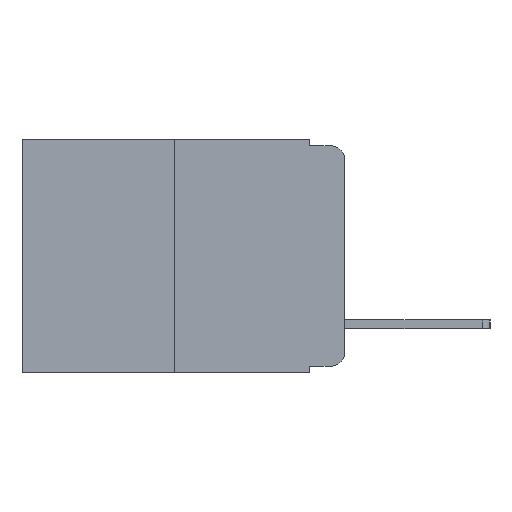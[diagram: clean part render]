
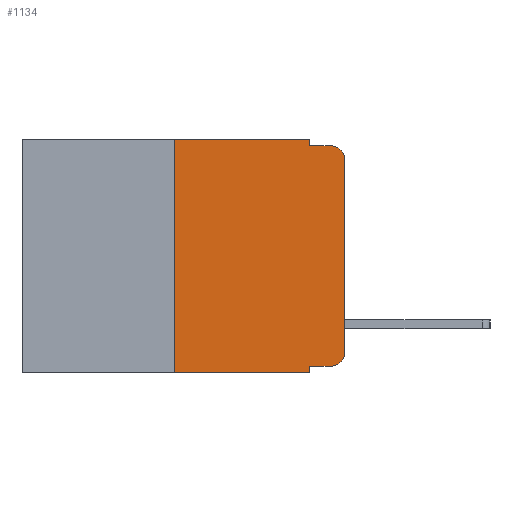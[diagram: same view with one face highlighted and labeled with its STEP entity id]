
A CAD part, left-side view. The second image highlights one B-rep face of the part: STEP entity #1134.
In plain terms, the highlighted planar face has unit normal (-1, 0, 0).
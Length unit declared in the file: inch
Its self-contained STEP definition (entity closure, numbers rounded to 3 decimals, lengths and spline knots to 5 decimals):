
#122 = EDGE_CURVE ( 'NONE', #4731, #6321, #10682, .T. ) ;
#1134 = ADVANCED_FACE ( 'NONE', ( #19873 ), #5024, .F. ) ;
#1407 = VECTOR ( 'NONE', #13175, 39.37008 ) ;
#1481 = LINE ( 'NONE', #19333, #18696 ) ;
#1490 = VECTOR ( 'NONE', #3155, 39.37008 ) ;
#1791 = DIRECTION ( 'NONE',  ( 0., 0., 1. ) ) ;
#1936 = EDGE_CURVE ( 'NONE', #8261, #8428, #20631, .T. ) ;
#2700 = CARTESIAN_POINT ( 'NONE',  ( 0., 0.051, 0. ) ) ;
#3056 = DIRECTION ( 'NONE',  ( 0., 0., -1. ) ) ;
#3059 = CARTESIAN_POINT ( 'NONE',  ( 0., 0.473, -0.343 ) ) ;
#3111 = DIRECTION ( 'NONE',  ( 1., 0., 0. ) ) ;
#3155 = DIRECTION ( 'NONE',  ( 0., 0., 1. ) ) ;
#3960 = DIRECTION ( 'NONE',  ( 0., 0., -1. ) ) ;
#4731 = VERTEX_POINT ( 'NONE', #2700 ) ;
#4747 = ORIENTED_EDGE ( 'NONE', *, *, #14317, .T. ) ;
#4881 = EDGE_LOOP ( 'NONE', ( #14698, #15232, #6627, #7158, #16296, #20698, #8278, #21745, #4747, #13901 ) ) ;
#4957 = CARTESIAN_POINT ( 'NONE',  ( 0., 0.051, -0.333 ) ) ;
#5024 = PLANE ( 'NONE',  #14241 ) ;
#5183 = DIRECTION ( 'NONE',  ( 0., -1., 0. ) ) ;
#6321 = VERTEX_POINT ( 'NONE', #17159 ) ;
#6346 = CARTESIAN_POINT ( 'NONE',  ( 0., 0.02, -0.03 ) ) ;
#6627 = ORIENTED_EDGE ( 'NONE', *, *, #8733, .F. ) ;
#6800 = CARTESIAN_POINT ( 'NONE',  ( 0., 0., -0.03 ) ) ;
#7158 = ORIENTED_EDGE ( 'NONE', *, *, #122, .F. ) ;
#8097 = DIRECTION ( 'NONE',  ( 0., 0., -1. ) ) ;
#8261 = VERTEX_POINT ( 'NONE', #16272 ) ;
#8278 = ORIENTED_EDGE ( 'NONE', *, *, #1936, .T. ) ;
#8428 = VERTEX_POINT ( 'NONE', #15004 ) ;
#8733 = EDGE_CURVE ( 'NONE', #6321, #12082, #14308, .T. ) ;
#8940 = DIRECTION ( 'NONE',  ( 0., -1., 0. ) ) ;
#9775 = VECTOR ( 'NONE', #8940, 39.37008 ) ;
#9841 = DIRECTION ( 'NONE',  ( -1., 0., 0. ) ) ;
#10122 = VECTOR ( 'NONE', #1791, 39.37008 ) ;
#10216 = VERTEX_POINT ( 'NONE', #14062 ) ;
#10307 = EDGE_CURVE ( 'NONE', #10216, #8428, #1481, .T. ) ;
#10682 = LINE ( 'NONE', #14152, #1407 ) ;
#10694 = EDGE_CURVE ( 'NONE', #12680, #15510, #19629, .T. ) ;
#11147 = AXIS2_PLACEMENT_3D ( 'NONE', #6346, #18289, #8097 ) ;
#11713 = VECTOR ( 'NONE', #16824, 39.37008 ) ;
#11892 = EDGE_CURVE ( 'NONE', #15510, #12082, #15130, .T. ) ;
#12080 = LINE ( 'NONE', #4957, #17106 ) ;
#12082 = VERTEX_POINT ( 'NONE', #22035 ) ;
#12345 = CARTESIAN_POINT ( 'NONE',  ( 0., 0.02, -0.333 ) ) ;
#12597 = VERTEX_POINT ( 'NONE', #12345 ) ;
#12680 = VERTEX_POINT ( 'NONE', #14269 ) ;
#13104 = VECTOR ( 'NONE', #5183, 39.37008 ) ;
#13175 = DIRECTION ( 'NONE',  ( 0., 0., -1. ) ) ;
#13437 = CIRCLE ( 'NONE', #22128, 0.02 ) ;
#13487 = CARTESIAN_POINT ( 'NONE',  ( 0., 0.25, 0. ) ) ;
#13601 = EDGE_CURVE ( 'NONE', #12597, #12680, #13437, .T. ) ;
#13727 = EDGE_CURVE ( 'NONE', #8261, #22092, #21290, .T. ) ;
#13901 = ORIENTED_EDGE ( 'NONE', *, *, #13601, .T. ) ;
#14062 = CARTESIAN_POINT ( 'NONE',  ( 0., 0.051, -0.333 ) ) ;
#14152 = CARTESIAN_POINT ( 'NONE',  ( 0., 0.051, 0. ) ) ;
#14169 = LINE ( 'NONE', #20426, #13104 ) ;
#14241 = AXIS2_PLACEMENT_3D ( 'NONE', #15697, #3111, #3056 ) ;
#14269 = CARTESIAN_POINT ( 'NONE',  ( 0., 0., -0.313 ) ) ;
#14308 = LINE ( 'NONE', #20673, #9775 ) ;
#14317 = EDGE_CURVE ( 'NONE', #10216, #12597, #12080, .T. ) ;
#14698 = ORIENTED_EDGE ( 'NONE', *, *, #10694, .T. ) ;
#15004 = CARTESIAN_POINT ( 'NONE',  ( 0., 0.051, -0.343 ) ) ;
#15130 = CIRCLE ( 'NONE', #11147, 0.02 ) ;
#15232 = ORIENTED_EDGE ( 'NONE', *, *, #11892, .T. ) ;
#15510 = VERTEX_POINT ( 'NONE', #6800 ) ;
#15697 = CARTESIAN_POINT ( 'NONE',  ( 0., 0.473, 0. ) ) ;
#16272 = CARTESIAN_POINT ( 'NONE',  ( 0., 0.25, -0.343 ) ) ;
#16296 = ORIENTED_EDGE ( 'NONE', *, *, #21825, .F. ) ;
#16824 = DIRECTION ( 'NONE',  ( 0., -1., 0. ) ) ;
#17106 = VECTOR ( 'NONE', #18628, 39.37008 ) ;
#17159 = CARTESIAN_POINT ( 'NONE',  ( 0., 0.051, -0.01 ) ) ;
#18289 = DIRECTION ( 'NONE',  ( -1., 0., 0. ) ) ;
#18628 = DIRECTION ( 'NONE',  ( 0., -1., 0. ) ) ;
#18696 = VECTOR ( 'NONE', #3960, 39.37008 ) ;
#19333 = CARTESIAN_POINT ( 'NONE',  ( 0., 0.051, 0. ) ) ;
#19407 = CARTESIAN_POINT ( 'NONE',  ( 0., 0.25, 0. ) ) ;
#19629 = LINE ( 'NONE', #22205, #10122 ) ;
#19873 = FACE_OUTER_BOUND ( 'NONE', #4881, .T. ) ;
#19951 = CARTESIAN_POINT ( 'NONE',  ( 0., 0.02, -0.313 ) ) ;
#20426 = CARTESIAN_POINT ( 'NONE',  ( 0., 0.473, 0. ) ) ;
#20631 = LINE ( 'NONE', #3059, #11713 ) ;
#20673 = CARTESIAN_POINT ( 'NONE',  ( 0., 0.051, -0.01 ) ) ;
#20698 = ORIENTED_EDGE ( 'NONE', *, *, #13727, .F. ) ;
#21290 = LINE ( 'NONE', #13487, #1490 ) ;
#21616 = DIRECTION ( 'NONE',  ( 0., 0., -1. ) ) ;
#21745 = ORIENTED_EDGE ( 'NONE', *, *, #10307, .F. ) ;
#21825 = EDGE_CURVE ( 'NONE', #22092, #4731, #14169, .T. ) ;
#22035 = CARTESIAN_POINT ( 'NONE',  ( 0., 0.02, -0.01 ) ) ;
#22092 = VERTEX_POINT ( 'NONE', #19407 ) ;
#22128 = AXIS2_PLACEMENT_3D ( 'NONE', #19951, #9841, #21616 ) ;
#22205 = CARTESIAN_POINT ( 'NONE',  ( 0., 0., 0. ) ) ;
